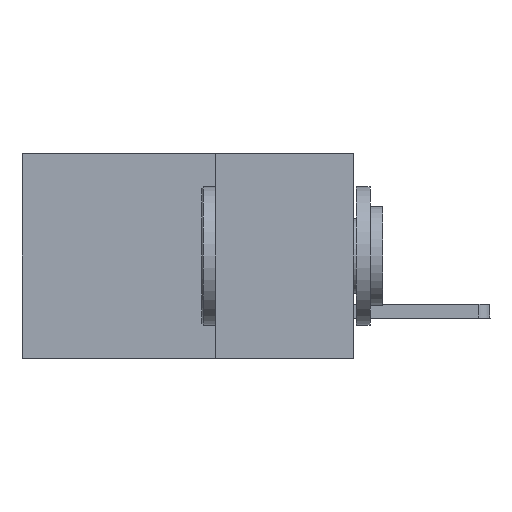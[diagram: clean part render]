
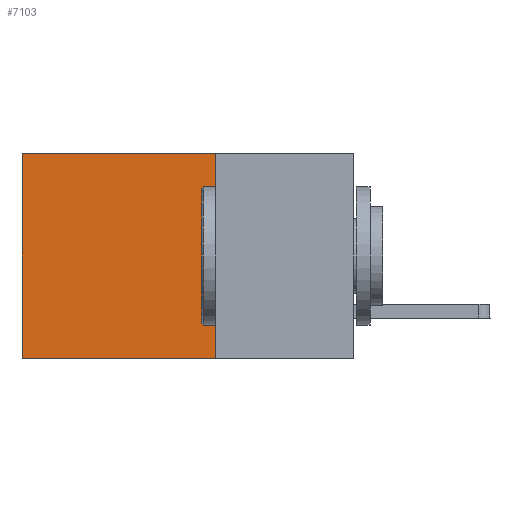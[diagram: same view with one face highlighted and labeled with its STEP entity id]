
A CAD part, left-side view. The second image highlights one B-rep face of the part: STEP entity #7103.
In plain terms, the highlighted planar face has unit normal (-1, 0, 0).
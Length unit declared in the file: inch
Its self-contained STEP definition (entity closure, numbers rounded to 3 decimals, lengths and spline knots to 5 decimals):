
#219 = EDGE_CURVE ( 'NONE', #5560, #1299, #1064, .T. ) ;
#724 = VERTEX_POINT ( 'NONE', #1469 ) ;
#1064 = LINE ( 'NONE', #4953, #12560 ) ;
#1126 = CARTESIAN_POINT ( 'NONE',  ( 0.2875, 0.25, 0. ) ) ;
#1299 = VERTEX_POINT ( 'NONE', #2764 ) ;
#1469 = CARTESIAN_POINT ( 'NONE',  ( 0.2875, 0.25, 0. ) ) ;
#1769 = LINE ( 'NONE', #11340, #3062 ) ;
#1964 = FACE_OUTER_BOUND ( 'NONE', #12751, .T. ) ;
#2514 = CARTESIAN_POINT ( 'NONE',  ( 0.2875, 0.6, 0. ) ) ;
#2744 = LINE ( 'NONE', #7611, #12246 ) ;
#2764 = CARTESIAN_POINT ( 'NONE',  ( 0.2875, 0.6, -0.37 ) ) ;
#3062 = VECTOR ( 'NONE', #5676, 39.37008 ) ;
#4112 = CARTESIAN_POINT ( 'NONE',  ( 0.2875, 0.25, 0. ) ) ;
#4436 = ORIENTED_EDGE ( 'NONE', *, *, #10181, .F. ) ;
#4953 = CARTESIAN_POINT ( 'NONE',  ( 0.2875, 0.25, -0.37 ) ) ;
#5560 = VERTEX_POINT ( 'NONE', #8548 ) ;
#5676 = DIRECTION ( 'NONE',  ( 0., 0., -1. ) ) ;
#5740 = DIRECTION ( 'NONE',  ( 1., 0., 0. ) ) ;
#5829 = DIRECTION ( 'NONE',  ( 0., 0., -1. ) ) ;
#5970 = LINE ( 'NONE', #4112, #12179 ) ;
#7103 = ADVANCED_FACE ( 'NONE', ( #1964 ), #9120, .F. ) ;
#7611 = CARTESIAN_POINT ( 'NONE',  ( 0.2875, 0.25, 0. ) ) ;
#7720 = VERTEX_POINT ( 'NONE', #2514 ) ;
#8058 = ORIENTED_EDGE ( 'NONE', *, *, #12166, .T. ) ;
#8548 = CARTESIAN_POINT ( 'NONE',  ( 0.2875, 0.25, -0.37 ) ) ;
#9120 = PLANE ( 'NONE',  #9983 ) ;
#9906 = DIRECTION ( 'NONE',  ( 0., 0., -1. ) ) ;
#9983 = AXIS2_PLACEMENT_3D ( 'NONE', #1126, #5740, #5829 ) ;
#10181 = EDGE_CURVE ( 'NONE', #724, #5560, #2744, .T. ) ;
#11266 = ORIENTED_EDGE ( 'NONE', *, *, #219, .F. ) ;
#11340 = CARTESIAN_POINT ( 'NONE',  ( 0.2875, 0.6, 0. ) ) ;
#11526 = ORIENTED_EDGE ( 'NONE', *, *, #11721, .T. ) ;
#11721 = EDGE_CURVE ( 'NONE', #7720, #1299, #1769, .T. ) ;
#11741 = DIRECTION ( 'NONE',  ( 0., 1., 0. ) ) ;
#12166 = EDGE_CURVE ( 'NONE', #724, #7720, #5970, .T. ) ;
#12179 = VECTOR ( 'NONE', #13438, 39.37008 ) ;
#12246 = VECTOR ( 'NONE', #9906, 39.37008 ) ;
#12560 = VECTOR ( 'NONE', #11741, 39.37008 ) ;
#12751 = EDGE_LOOP ( 'NONE', ( #11526, #11266, #4436, #8058 ) ) ;
#13438 = DIRECTION ( 'NONE',  ( 0., 1., 0. ) ) ;
